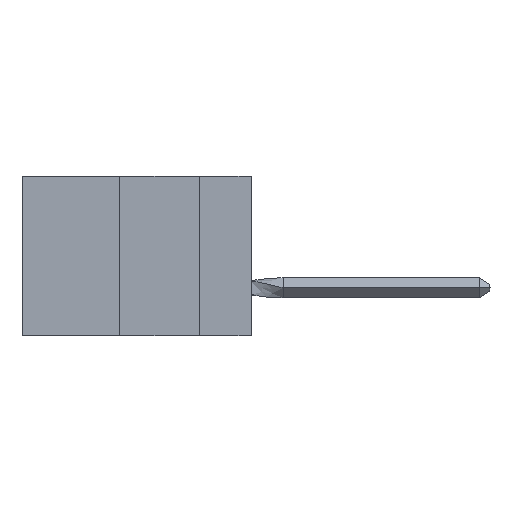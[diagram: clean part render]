
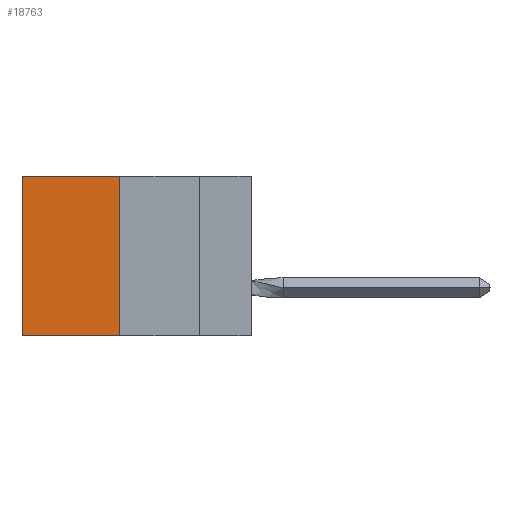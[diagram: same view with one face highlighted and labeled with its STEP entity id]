
A CAD part, left-side view. The second image highlights one B-rep face of the part: STEP entity #18763.
In plain terms, the highlighted planar face has unit normal (-1, 0, 0).
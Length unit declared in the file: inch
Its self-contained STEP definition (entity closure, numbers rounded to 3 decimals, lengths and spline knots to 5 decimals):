
#228 = VERTEX_POINT ( 'NONE', #19445 ) ;
#656 = DIRECTION ( 'NONE',  ( 1., 0., 0. ) ) ;
#1449 = VECTOR ( 'NONE', #14995, 39.37008 ) ;
#1926 = VECTOR ( 'NONE', #19455, 39.37008 ) ;
#4605 = AXIS2_PLACEMENT_3D ( 'NONE', #17636, #656, #13209 ) ;
#5451 = CARTESIAN_POINT ( 'NONE',  ( 0.305, 0.413, 0. ) ) ;
#5459 = CARTESIAN_POINT ( 'NONE',  ( 0.305, 0.413, -0.5 ) ) ;
#5548 = CARTESIAN_POINT ( 'NONE',  ( 0.305, 0.413, -0.5 ) ) ;
#5894 = EDGE_CURVE ( 'NONE', #16429, #11804, #15188, .T. ) ;
#6136 = CARTESIAN_POINT ( 'NONE',  ( 0.305, 0.413, -0.5 ) ) ;
#6674 = DIRECTION ( 'NONE',  ( 0., 1., 0. ) ) ;
#6940 = PLANE ( 'NONE',  #4605 ) ;
#8168 = CARTESIAN_POINT ( 'NONE',  ( 0.305, 0.413, 0. ) ) ;
#9715 = EDGE_LOOP ( 'NONE', ( #9789, #12324, #9922, #18496 ) ) ;
#9778 = CARTESIAN_POINT ( 'NONE',  ( 0.305, 0.72, 0. ) ) ;
#9789 = ORIENTED_EDGE ( 'NONE', *, *, #17027, .T. ) ;
#9922 = ORIENTED_EDGE ( 'NONE', *, *, #5894, .F. ) ;
#9964 = EDGE_CURVE ( 'NONE', #11804, #228, #15781, .T. ) ;
#10163 = LINE ( 'NONE', #8168, #17871 ) ;
#10857 = EDGE_CURVE ( 'NONE', #16429, #17608, #10163, .T. ) ;
#11804 = VERTEX_POINT ( 'NONE', #5548 ) ;
#12324 = ORIENTED_EDGE ( 'NONE', *, *, #9964, .F. ) ;
#13209 = DIRECTION ( 'NONE',  ( 0., 0., -1. ) ) ;
#13239 = VECTOR ( 'NONE', #16900, 39.37008 ) ;
#13271 = CARTESIAN_POINT ( 'NONE',  ( 0.305, 0.72, -0.5 ) ) ;
#14995 = DIRECTION ( 'NONE',  ( 0., 1., 0. ) ) ;
#15055 = LINE ( 'NONE', #13271, #1926 ) ;
#15188 = LINE ( 'NONE', #6136, #13239 ) ;
#15781 = LINE ( 'NONE', #5459, #1449 ) ;
#16429 = VERTEX_POINT ( 'NONE', #5451 ) ;
#16900 = DIRECTION ( 'NONE',  ( 0., 0., -1. ) ) ;
#17027 = EDGE_CURVE ( 'NONE', #17608, #228, #15055, .T. ) ;
#17608 = VERTEX_POINT ( 'NONE', #9778 ) ;
#17609 = FACE_OUTER_BOUND ( 'NONE', #9715, .T. ) ;
#17636 = CARTESIAN_POINT ( 'NONE',  ( 0.305, 0.413, -0.5 ) ) ;
#17871 = VECTOR ( 'NONE', #6674, 39.37008 ) ;
#18496 = ORIENTED_EDGE ( 'NONE', *, *, #10857, .T. ) ;
#18763 = ADVANCED_FACE ( 'NONE', ( #17609 ), #6940, .F. ) ;
#19445 = CARTESIAN_POINT ( 'NONE',  ( 0.305, 0.72, -0.5 ) ) ;
#19455 = DIRECTION ( 'NONE',  ( 0., 0., -1. ) ) ;
